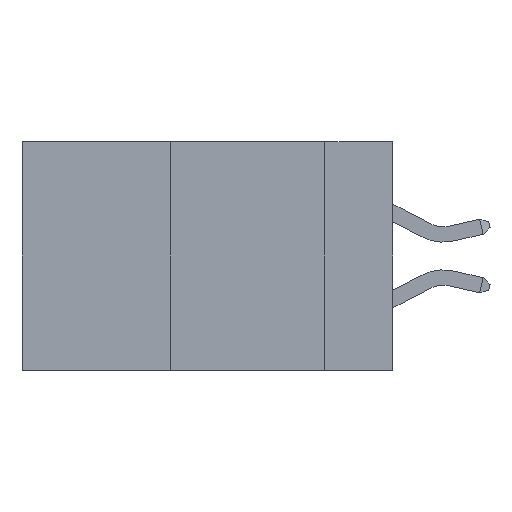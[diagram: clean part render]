
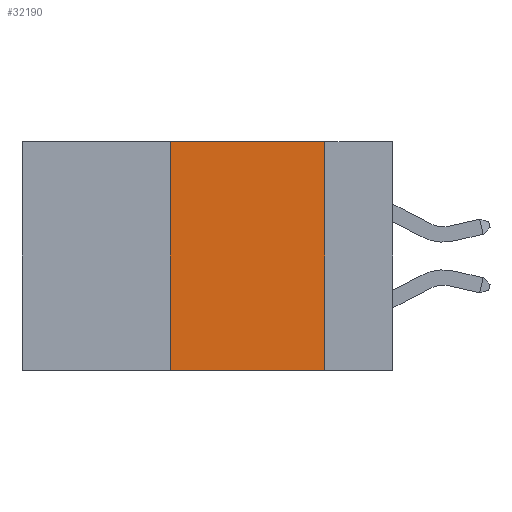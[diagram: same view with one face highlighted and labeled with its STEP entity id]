
A CAD part, left-side view. The second image highlights one B-rep face of the part: STEP entity #32190.
In plain terms, the highlighted planar face has unit normal (-1, 0, 0).
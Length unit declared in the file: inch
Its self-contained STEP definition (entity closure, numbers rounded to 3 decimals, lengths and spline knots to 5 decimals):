
#7 = VERTEX_POINT ( 'NONE', #35007 ) ;
#646 = DIRECTION ( 'NONE',  ( 0., -1., 0. ) ) ;
#2443 = CARTESIAN_POINT ( 'NONE',  ( 0., 0.36, -0.37 ) ) ;
#2905 = LINE ( 'NONE', #35189, #24421 ) ;
#4196 = DIRECTION ( 'NONE',  ( 0., 0., -1. ) ) ;
#4490 = ORIENTED_EDGE ( 'NONE', *, *, #14096, .F. ) ;
#5608 = VERTEX_POINT ( 'NONE', #5799 ) ;
#5776 = AXIS2_PLACEMENT_3D ( 'NONE', #18854, #27892, #25107 ) ;
#5799 = CARTESIAN_POINT ( 'NONE',  ( 0., 0.11, 0. ) ) ;
#8867 = FACE_OUTER_BOUND ( 'NONE', #33452, .T. ) ;
#9511 = LINE ( 'NONE', #33246, #15000 ) ;
#10431 = PLANE ( 'NONE',  #5776 ) ;
#11585 = DIRECTION ( 'NONE',  ( 0., -1., 0. ) ) ;
#14096 = EDGE_CURVE ( 'NONE', #7, #5608, #2905, .T. ) ;
#15000 = VECTOR ( 'NONE', #4196, 39.37008 ) ;
#17549 = EDGE_CURVE ( 'NONE', #5608, #22292, #9511, .T. ) ;
#18854 = CARTESIAN_POINT ( 'NONE',  ( 0., 0.6, 0. ) ) ;
#19243 = LINE ( 'NONE', #31123, #31586 ) ;
#19509 = DIRECTION ( 'NONE',  ( 0., 0., 1. ) ) ;
#20169 = LINE ( 'NONE', #29559, #25186 ) ;
#20367 = VERTEX_POINT ( 'NONE', #2443 ) ;
#22292 = VERTEX_POINT ( 'NONE', #23234 ) ;
#23234 = CARTESIAN_POINT ( 'NONE',  ( 0., 0.11, -0.37 ) ) ;
#24421 = VECTOR ( 'NONE', #11585, 39.37008 ) ;
#25107 = DIRECTION ( 'NONE',  ( 0., 0., -1. ) ) ;
#25186 = VECTOR ( 'NONE', #646, 39.37008 ) ;
#26419 = EDGE_CURVE ( 'NONE', #20367, #7, #19243, .T. ) ;
#26694 = EDGE_CURVE ( 'NONE', #20367, #22292, #20169, .T. ) ;
#27892 = DIRECTION ( 'NONE',  ( 1., 0., 0. ) ) ;
#28029 = ORIENTED_EDGE ( 'NONE', *, *, #26694, .T. ) ;
#29404 = ORIENTED_EDGE ( 'NONE', *, *, #26419, .F. ) ;
#29559 = CARTESIAN_POINT ( 'NONE',  ( 0., 0.6, -0.37 ) ) ;
#30227 = ORIENTED_EDGE ( 'NONE', *, *, #17549, .F. ) ;
#31123 = CARTESIAN_POINT ( 'NONE',  ( 0., 0.36, 0. ) ) ;
#31586 = VECTOR ( 'NONE', #19509, 39.37008 ) ;
#32190 = ADVANCED_FACE ( 'NONE', ( #8867 ), #10431, .F. ) ;
#33246 = CARTESIAN_POINT ( 'NONE',  ( 0., 0.11, 0. ) ) ;
#33452 = EDGE_LOOP ( 'NONE', ( #30227, #4490, #29404, #28029 ) ) ;
#35007 = CARTESIAN_POINT ( 'NONE',  ( 0., 0.36, 0. ) ) ;
#35189 = CARTESIAN_POINT ( 'NONE',  ( 0., 0.6, 0. ) ) ;
